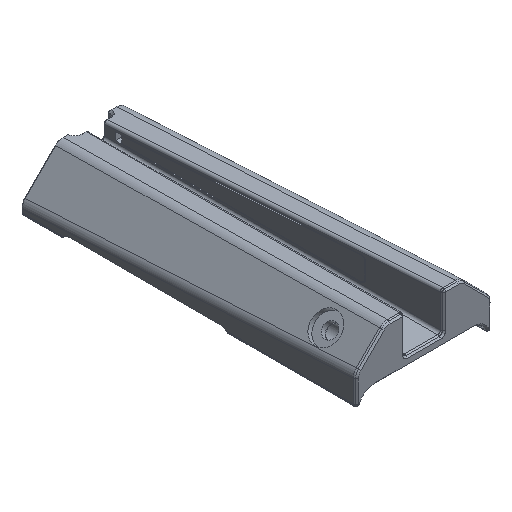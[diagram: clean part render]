
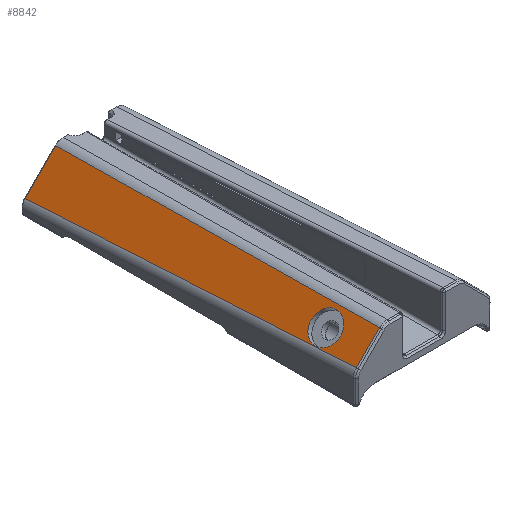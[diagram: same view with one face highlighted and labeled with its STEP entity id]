
A CAD part, isometric view. The second image highlights one B-rep face of the part: STEP entity #8842.
In plain terms, the highlighted planar face has unit normal (-0.707, 0.04, 0.706).
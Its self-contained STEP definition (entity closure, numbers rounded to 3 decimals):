
#23=FACE_BOUND('',#2704,.T.);
#80=ELLIPSE('',#9528,2.802,2.8);
#230=PLANE('',#9596);
#695=LINE('',#14151,#1353);
#738=LINE('',#14962,#1396);
#739=LINE('',#14970,#1397);
#740=LINE('',#14971,#1398);
#1353=VECTOR('',#11070,10.);
#1396=VECTOR('',#11195,10.);
#1397=VECTOR('',#11198,10.);
#1398=VECTOR('',#11199,10.);
#2139=FACE_OUTER_BOUND('',#2703,.T.);
#2703=EDGE_LOOP('',(#6957,#6958,#6959,#6960,#6961,#6962,#6963));
#2704=EDGE_LOOP('',(#6964));
#3390=B_SPLINE_CURVE_WITH_KNOTS('',3,(#14137,#14138,#14139,#14140),
 .UNSPECIFIED.,.F.,.F.,(4,4),(0.,0.001),.UNSPECIFIED.);
#3392=B_SPLINE_CURVE_WITH_KNOTS('',3,(#14169,#14170,#14171,#14172),
 .UNSPECIFIED.,.F.,.F.,(4,4),(0.,0.001),
 .UNSPECIFIED.);
#3437=B_SPLINE_CURVE_WITH_KNOTS('',3,(#14965,#14966,#14967,#14968),
 .UNSPECIFIED.,.F.,.F.,(4,4),(0.218,0.22),
 .UNSPECIFIED.);
#3909=VERTEX_POINT('',#14006);
#3927=VERTEX_POINT('',#14093);
#3928=VERTEX_POINT('',#14133);
#3930=VERTEX_POINT('',#14136);
#3932=VERTEX_POINT('',#14148);
#4001=VERTEX_POINT('',#14957);
#4002=VERTEX_POINT('',#14964);
#4003=VERTEX_POINT('',#14969);
#4911=EDGE_CURVE('',#3909,#3909,#80,.T.);
#4938=EDGE_CURVE('',#3930,#3928,#3390,.T.);
#4942=EDGE_CURVE('',#3928,#3932,#695,.T.);
#4944=EDGE_CURVE('',#3927,#3930,#3392,.T.);
#5056=EDGE_CURVE('',#3932,#4001,#738,.T.);
#5057=EDGE_CURVE('',#4001,#4002,#3437,.T.);
#5058=EDGE_CURVE('',#4002,#4003,#739,.T.);
#5059=EDGE_CURVE('',#4003,#3927,#740,.T.);
#6957=ORIENTED_EDGE('',*,*,#4944,.T.);
#6958=ORIENTED_EDGE('',*,*,#4938,.T.);
#6959=ORIENTED_EDGE('',*,*,#4942,.T.);
#6960=ORIENTED_EDGE('',*,*,#5056,.T.);
#6961=ORIENTED_EDGE('',*,*,#5057,.T.);
#6962=ORIENTED_EDGE('',*,*,#5058,.T.);
#6963=ORIENTED_EDGE('',*,*,#5059,.T.);
#6964=ORIENTED_EDGE('',*,*,#4911,.F.);
#8842=ADVANCED_FACE('',(#2139,#23),#230,.T.);
#9528=AXIS2_PLACEMENT_3D('',#14008,#11012,#11013);
#9596=AXIS2_PLACEMENT_3D('',#14963,#11196,#11197);
#11012=DIRECTION('center_axis',(-0.707,0.04,0.706));
#11013=DIRECTION('ref_axis',(0.026,0.999,-0.032));
#11070=DIRECTION('',(0.707,0.,0.707));
#11195=DIRECTION('',(0.022,0.999,-0.035));
#11196=DIRECTION('center_axis',(-0.707,0.04,0.706));
#11197=DIRECTION('ref_axis',(0.707,0.,0.707));
#11198=DIRECTION('',(-0.707,0.,-0.707));
#11199=DIRECTION('',(0.,-0.998,0.057));
#14006=CARTESIAN_POINT('',(-10.193,-0.028,7.825));
#14008=CARTESIAN_POINT('Origin',(-10.113,2.772,7.745));
#14093=CARTESIAN_POINT('',(-12.163,-4.991,6.137));
#14133=CARTESIAN_POINT('',(-12.147,-4.991,6.154));
#14136=CARTESIAN_POINT('',(-12.157,-4.991,6.143));
#14137=CARTESIAN_POINT('Ctrl Pts',(-12.157,-4.991,
6.143));
#14138=CARTESIAN_POINT('Ctrl Pts',(-12.154,-4.991,
6.147));
#14139=CARTESIAN_POINT('Ctrl Pts',(-12.15,-4.991,6.15));
#14140=CARTESIAN_POINT('Ctrl Pts',(-12.147,-4.991,
6.154));
#14148=CARTESIAN_POINT('',(-7.791,-4.991,10.511));
#14151=CARTESIAN_POINT('',(-10.472,-4.991,7.83));
#14169=CARTESIAN_POINT('Ctrl Pts',(-12.163,-4.991,
6.137));
#14170=CARTESIAN_POINT('Ctrl Pts',(-12.161,-4.991,
6.139));
#14171=CARTESIAN_POINT('Ctrl Pts',(-12.159,-4.991,
6.141));
#14172=CARTESIAN_POINT('Ctrl Pts',(-12.157,-4.991,
6.143));
#14957=CARTESIAN_POINT('',(-6.415,57.139,8.342));
#14962=CARTESIAN_POINT('',(-7.008,30.376,9.276));
#14963=CARTESIAN_POINT('Origin',(-10.06,30.369,6.223));
#14964=CARTESIAN_POINT('',(-6.417,57.139,8.339));
#14965=CARTESIAN_POINT('Ctrl Pts',(-6.415,57.139,8.342));
#14966=CARTESIAN_POINT('Ctrl Pts',(-6.416,57.139,8.341));
#14967=CARTESIAN_POINT('Ctrl Pts',(-6.417,57.139,8.34));
#14968=CARTESIAN_POINT('Ctrl Pts',(-6.417,57.139,8.339));
#14969=CARTESIAN_POINT('',(-12.163,57.139,2.591));
#14970=CARTESIAN_POINT('',(-7.338,57.139,7.419));
#14971=CARTESIAN_POINT('',(-12.163,30.805,4.094));
